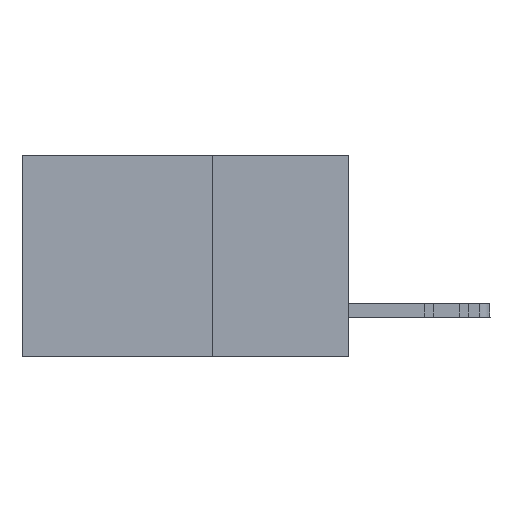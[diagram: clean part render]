
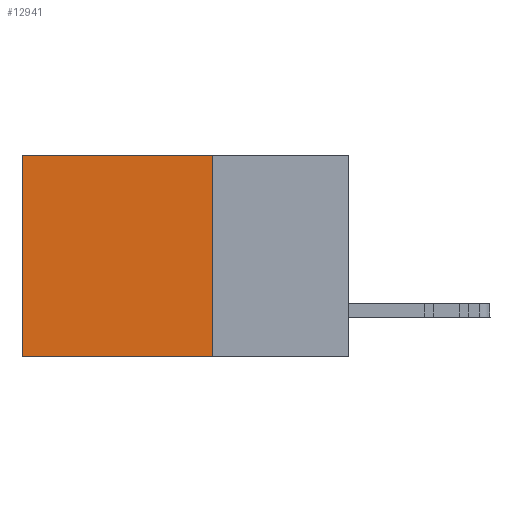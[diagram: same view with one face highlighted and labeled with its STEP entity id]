
A CAD part, left-side view. The second image highlights one B-rep face of the part: STEP entity #12941.
In plain terms, the highlighted planar face has unit normal (-1, 0, 0).
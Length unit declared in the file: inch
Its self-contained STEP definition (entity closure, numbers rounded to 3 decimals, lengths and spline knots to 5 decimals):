
#287 = CARTESIAN_POINT ( 'NONE',  ( 0.298, 0.25, 0. ) ) ;
#1872 = EDGE_CURVE ( 'NONE', #25815, #20629, #11529, .T. ) ;
#2008 = DIRECTION ( 'NONE',  ( 0., 0., -1. ) ) ;
#2953 = LINE ( 'NONE', #4140, #27781 ) ;
#3440 = CARTESIAN_POINT ( 'NONE',  ( 0.298, 0.6, 0. ) ) ;
#3537 = CARTESIAN_POINT ( 'NONE',  ( 0.298, 0.25, 0. ) ) ;
#4140 = CARTESIAN_POINT ( 'NONE',  ( 0.298, 0.25, 0. ) ) ;
#4189 = ORIENTED_EDGE ( 'NONE', *, *, #17805, .T. ) ;
#4224 = VECTOR ( 'NONE', #24505, 39.37008 ) ;
#5745 = CARTESIAN_POINT ( 'NONE',  ( 0.298, 0.6, 0. ) ) ;
#6419 = FACE_OUTER_BOUND ( 'NONE', #20429, .T. ) ;
#8226 = EDGE_CURVE ( 'NONE', #17219, #25815, #2953, .T. ) ;
#8411 = DIRECTION ( 'NONE',  ( 0., 0., -1. ) ) ;
#11529 = LINE ( 'NONE', #24391, #22748 ) ;
#11766 = VECTOR ( 'NONE', #8411, 39.37008 ) ;
#12941 = ADVANCED_FACE ( 'NONE', ( #6419 ), #13500, .F. ) ;
#13500 = PLANE ( 'NONE',  #21371 ) ;
#14634 = VERTEX_POINT ( 'NONE', #5745 ) ;
#17219 = VERTEX_POINT ( 'NONE', #3537 ) ;
#17295 = DIRECTION ( 'NONE',  ( 0., 1., 0. ) ) ;
#17805 = EDGE_CURVE ( 'NONE', #14634, #20629, #24501, .T. ) ;
#20060 = CARTESIAN_POINT ( 'NONE',  ( 0.298, 0.6, -0.37 ) ) ;
#20429 = EDGE_LOOP ( 'NONE', ( #4189, #26875, #24624, #29120 ) ) ;
#20629 = VERTEX_POINT ( 'NONE', #20060 ) ;
#21148 = CARTESIAN_POINT ( 'NONE',  ( 0.298, 0.25, 0. ) ) ;
#21305 = EDGE_CURVE ( 'NONE', #17219, #14634, #26837, .T. ) ;
#21371 = AXIS2_PLACEMENT_3D ( 'NONE', #21148, #30367, #2008 ) ;
#22748 = VECTOR ( 'NONE', #17295, 39.37008 ) ;
#24391 = CARTESIAN_POINT ( 'NONE',  ( 0.298, 0.25, -0.37 ) ) ;
#24501 = LINE ( 'NONE', #3440, #11766 ) ;
#24505 = DIRECTION ( 'NONE',  ( 0., 1., 0. ) ) ;
#24624 = ORIENTED_EDGE ( 'NONE', *, *, #8226, .F. ) ;
#25815 = VERTEX_POINT ( 'NONE', #29084 ) ;
#25816 = DIRECTION ( 'NONE',  ( 0., 0., -1. ) ) ;
#26837 = LINE ( 'NONE', #287, #4224 ) ;
#26875 = ORIENTED_EDGE ( 'NONE', *, *, #1872, .F. ) ;
#27781 = VECTOR ( 'NONE', #25816, 39.37008 ) ;
#29084 = CARTESIAN_POINT ( 'NONE',  ( 0.298, 0.25, -0.37 ) ) ;
#29120 = ORIENTED_EDGE ( 'NONE', *, *, #21305, .T. ) ;
#30367 = DIRECTION ( 'NONE',  ( 1., 0., 0. ) ) ;
